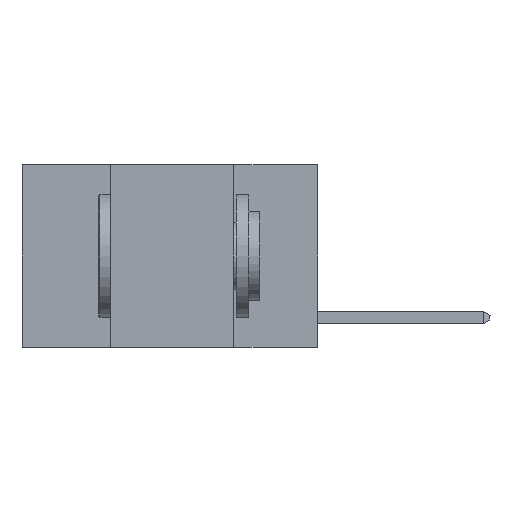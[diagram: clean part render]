
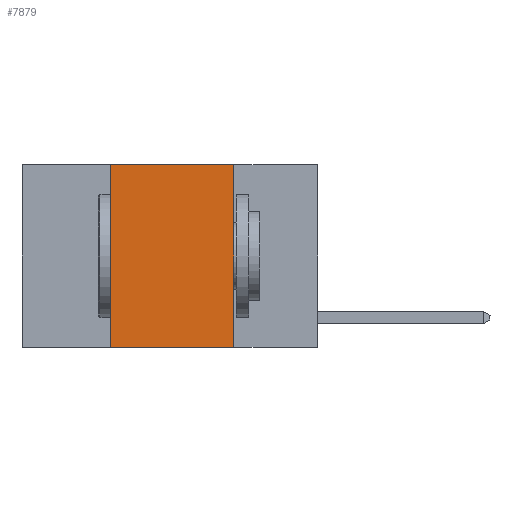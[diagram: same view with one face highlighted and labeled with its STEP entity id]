
A CAD part, left-side view. The second image highlights one B-rep face of the part: STEP entity #7879.
In plain terms, the highlighted planar face has unit normal (-1, 0, 0).
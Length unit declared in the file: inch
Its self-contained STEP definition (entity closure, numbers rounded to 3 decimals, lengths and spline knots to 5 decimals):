
#174 = VERTEX_POINT ( 'NONE', #12989 ) ;
#446 = DIRECTION ( 'NONE',  ( 1., 0., 0. ) ) ;
#504 = DIRECTION ( 'NONE',  ( 0., -1., 0. ) ) ;
#561 = CARTESIAN_POINT ( 'NONE',  ( 0., 0.17, 0. ) ) ;
#1122 = FACE_OUTER_BOUND ( 'NONE', #13392, .T. ) ;
#1341 = VECTOR ( 'NONE', #2690, 39.37008 ) ;
#2051 = VECTOR ( 'NONE', #504, 39.37008 ) ;
#2187 = PLANE ( 'NONE',  #16639 ) ;
#2690 = DIRECTION ( 'NONE',  ( 0., 0., 1. ) ) ;
#2723 = LINE ( 'NONE', #11253, #22307 ) ;
#3395 = CARTESIAN_POINT ( 'NONE',  ( 0., 0.42, 0. ) ) ;
#3738 = EDGE_CURVE ( 'NONE', #11025, #174, #5379, .T. ) ;
#4058 = EDGE_CURVE ( 'NONE', #11025, #12053, #9369, .T. ) ;
#4223 = DIRECTION ( 'NONE',  ( 0., 0., -1. ) ) ;
#5379 = LINE ( 'NONE', #19843, #2051 ) ;
#5438 = CARTESIAN_POINT ( 'NONE',  ( 0., 0.6, 0. ) ) ;
#5602 = CARTESIAN_POINT ( 'NONE',  ( 0., 0.6, 0. ) ) ;
#5853 = ORIENTED_EDGE ( 'NONE', *, *, #4058, .F. ) ;
#7000 = EDGE_CURVE ( 'NONE', #12053, #15551, #14387, .T. ) ;
#7118 = ORIENTED_EDGE ( 'NONE', *, *, #3738, .T. ) ;
#7879 = ADVANCED_FACE ( 'NONE', ( #1122 ), #2187, .F. ) ;
#8083 = ORIENTED_EDGE ( 'NONE', *, *, #19929, .F. ) ;
#9369 = LINE ( 'NONE', #13197, #1341 ) ;
#11025 = VERTEX_POINT ( 'NONE', #16152 ) ;
#11253 = CARTESIAN_POINT ( 'NONE',  ( 0., 0.17, 0. ) ) ;
#12053 = VERTEX_POINT ( 'NONE', #3395 ) ;
#12525 = ORIENTED_EDGE ( 'NONE', *, *, #7000, .F. ) ;
#12642 = DIRECTION ( 'NONE',  ( 0., -1., 0. ) ) ;
#12989 = CARTESIAN_POINT ( 'NONE',  ( 0., 0.17, -0.37 ) ) ;
#13197 = CARTESIAN_POINT ( 'NONE',  ( 0., 0.42, 0. ) ) ;
#13392 = EDGE_LOOP ( 'NONE', ( #8083, #12525, #5853, #7118 ) ) ;
#14387 = LINE ( 'NONE', #5602, #16950 ) ;
#15551 = VERTEX_POINT ( 'NONE', #561 ) ;
#16122 = DIRECTION ( 'NONE',  ( 0., 0., -1. ) ) ;
#16152 = CARTESIAN_POINT ( 'NONE',  ( 0., 0.42, -0.37 ) ) ;
#16639 = AXIS2_PLACEMENT_3D ( 'NONE', #5438, #446, #16122 ) ;
#16950 = VECTOR ( 'NONE', #12642, 39.37008 ) ;
#19843 = CARTESIAN_POINT ( 'NONE',  ( 0., 0.6, -0.37 ) ) ;
#19929 = EDGE_CURVE ( 'NONE', #15551, #174, #2723, .T. ) ;
#22307 = VECTOR ( 'NONE', #4223, 39.37008 ) ;
